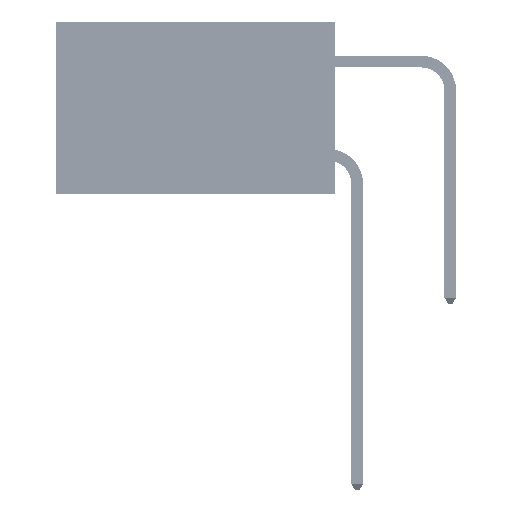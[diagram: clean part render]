
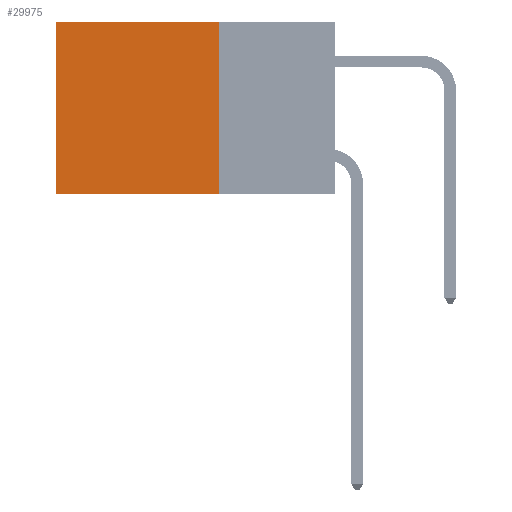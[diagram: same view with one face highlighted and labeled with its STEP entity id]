
A CAD part, left-side view. The second image highlights one B-rep face of the part: STEP entity #29975.
In plain terms, the highlighted planar face has unit normal (-1, 0, 0).
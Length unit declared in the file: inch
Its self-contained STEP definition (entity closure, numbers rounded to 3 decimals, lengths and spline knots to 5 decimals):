
#10 = CARTESIAN_POINT ( 'NONE',  ( 0.2875, 0.25, 0. ) ) ;
#417 = EDGE_CURVE ( 'NONE', #10934, #26075, #42224, .T. ) ;
#3074 = PLANE ( 'NONE',  #39097 ) ;
#3246 = DIRECTION ( 'NONE',  ( 0., 0., -1. ) ) ;
#4065 = VECTOR ( 'NONE', #3246, 39.37008 ) ;
#4593 = CARTESIAN_POINT ( 'NONE',  ( 0.2875, 0.25, 0. ) ) ;
#5596 = VECTOR ( 'NONE', #34815, 39.37008 ) ;
#6578 = DIRECTION ( 'NONE',  ( 0., 0., -1. ) ) ;
#7192 = CARTESIAN_POINT ( 'NONE',  ( 0.2875, 0.25, 0. ) ) ;
#7506 = CARTESIAN_POINT ( 'NONE',  ( 0.2875, 0.25, -0.37 ) ) ;
#9535 = EDGE_CURVE ( 'NONE', #10934, #23527, #19880, .T. ) ;
#10243 = DIRECTION ( 'NONE',  ( 1., 0., 0. ) ) ;
#10934 = VERTEX_POINT ( 'NONE', #7192 ) ;
#11524 = VECTOR ( 'NONE', #34196, 39.37008 ) ;
#14804 = ORIENTED_EDGE ( 'NONE', *, *, #9535, .T. ) ;
#17304 = EDGE_LOOP ( 'NONE', ( #19290, #49253, #45400, #14804 ) ) ;
#18444 = VERTEX_POINT ( 'NONE', #29123 ) ;
#19290 = ORIENTED_EDGE ( 'NONE', *, *, #30055, .T. ) ;
#19880 = LINE ( 'NONE', #4593, #5596 ) ;
#21748 = CARTESIAN_POINT ( 'NONE',  ( 0.2875, 0.25, 0. ) ) ;
#23527 = VERTEX_POINT ( 'NONE', #23829 ) ;
#23829 = CARTESIAN_POINT ( 'NONE',  ( 0.2875, 0.6, 0. ) ) ;
#26075 = VERTEX_POINT ( 'NONE', #37194 ) ;
#29123 = CARTESIAN_POINT ( 'NONE',  ( 0.2875, 0.6, -0.37 ) ) ;
#29975 = ADVANCED_FACE ( 'NONE', ( #41658 ), #3074, .F. ) ;
#30053 = LINE ( 'NONE', #7506, #11524 ) ;
#30055 = EDGE_CURVE ( 'NONE', #23527, #18444, #39263, .T. ) ;
#34196 = DIRECTION ( 'NONE',  ( 0., 1., 0. ) ) ;
#34815 = DIRECTION ( 'NONE',  ( 0., 1., 0. ) ) ;
#37045 = EDGE_CURVE ( 'NONE', #26075, #18444, #30053, .T. ) ;
#37194 = CARTESIAN_POINT ( 'NONE',  ( 0.2875, 0.25, -0.37 ) ) ;
#38199 = DIRECTION ( 'NONE',  ( 0., 0., -1. ) ) ;
#39097 = AXIS2_PLACEMENT_3D ( 'NONE', #21748, #10243, #6578 ) ;
#39263 = LINE ( 'NONE', #45965, #4065 ) ;
#41658 = FACE_OUTER_BOUND ( 'NONE', #17304, .T. ) ;
#42224 = LINE ( 'NONE', #10, #45857 ) ;
#45400 = ORIENTED_EDGE ( 'NONE', *, *, #417, .F. ) ;
#45857 = VECTOR ( 'NONE', #38199, 39.37008 ) ;
#45965 = CARTESIAN_POINT ( 'NONE',  ( 0.2875, 0.6, 0. ) ) ;
#49253 = ORIENTED_EDGE ( 'NONE', *, *, #37045, .F. ) ;
